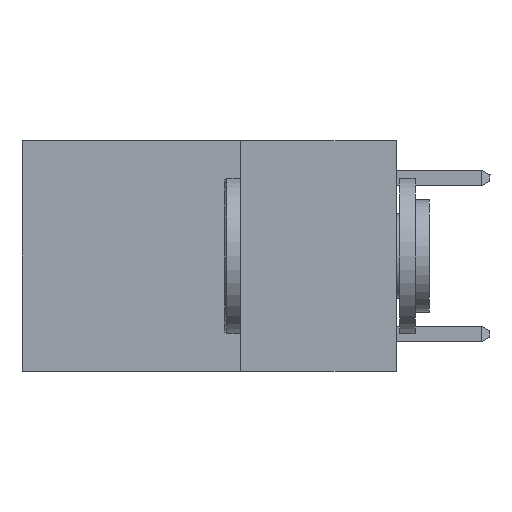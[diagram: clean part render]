
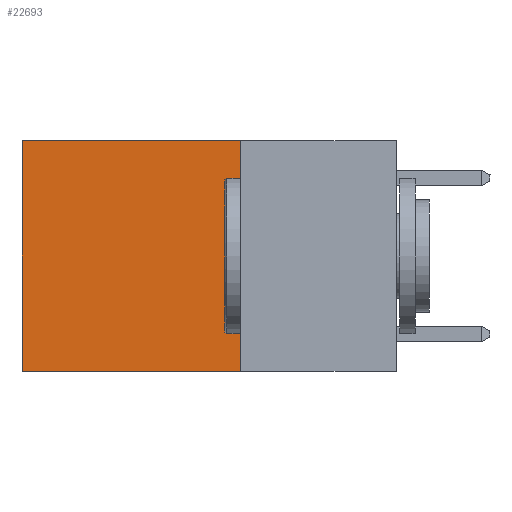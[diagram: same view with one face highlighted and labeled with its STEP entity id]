
A CAD part, left-side view. The second image highlights one B-rep face of the part: STEP entity #22693.
In plain terms, the highlighted planar face has unit normal (-1, 0, 0).
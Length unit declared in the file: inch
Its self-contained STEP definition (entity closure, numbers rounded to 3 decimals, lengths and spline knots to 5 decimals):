
#64 = LINE ( 'NONE', #23165, #13467 ) ;
#494 = LINE ( 'NONE', #6190, #6192 ) ;
#1434 = DIRECTION ( 'NONE',  ( 1., 0., 0. ) ) ;
#1438 = CARTESIAN_POINT ( 'NONE',  ( 0.2625, 0.25, -0.37 ) ) ;
#2534 = EDGE_LOOP ( 'NONE', ( #8610, #15364, #21157, #10491 ) ) ;
#2859 = PLANE ( 'NONE',  #4128 ) ;
#3209 = CARTESIAN_POINT ( 'NONE',  ( 0.2625, 0.25, 0. ) ) ;
#3812 = LINE ( 'NONE', #18160, #12394 ) ;
#4128 = AXIS2_PLACEMENT_3D ( 'NONE', #3209, #1434, #8187 ) ;
#6190 = CARTESIAN_POINT ( 'NONE',  ( 0.2625, 0.25, 0. ) ) ;
#6192 = VECTOR ( 'NONE', #16680, 39.37008 ) ;
#7245 = DIRECTION ( 'NONE',  ( 0., 1., 0. ) ) ;
#7482 = EDGE_CURVE ( 'NONE', #9780, #17205, #17042, .T. ) ;
#8187 = DIRECTION ( 'NONE',  ( 0., 0., -1. ) ) ;
#8610 = ORIENTED_EDGE ( 'NONE', *, *, #7482, .T. ) ;
#9780 = VERTEX_POINT ( 'NONE', #21618 ) ;
#10418 = FACE_OUTER_BOUND ( 'NONE', #2534, .T. ) ;
#10491 = ORIENTED_EDGE ( 'NONE', *, *, #22765, .T. ) ;
#11416 = CARTESIAN_POINT ( 'NONE',  ( 0.2625, 0.6, 0. ) ) ;
#12394 = VECTOR ( 'NONE', #7245, 39.37008 ) ;
#13327 = EDGE_CURVE ( 'NONE', #20105, #13596, #494, .T. ) ;
#13467 = VECTOR ( 'NONE', #19700, 39.37008 ) ;
#13541 = CARTESIAN_POINT ( 'NONE',  ( 0.2625, 0.6, -0.37 ) ) ;
#13596 = VERTEX_POINT ( 'NONE', #1438 ) ;
#15364 = ORIENTED_EDGE ( 'NONE', *, *, #22854, .F. ) ;
#16579 = VECTOR ( 'NONE', #16937, 39.37008 ) ;
#16680 = DIRECTION ( 'NONE',  ( 0., 0., -1. ) ) ;
#16937 = DIRECTION ( 'NONE',  ( 0., 0., -1. ) ) ;
#17042 = LINE ( 'NONE', #11416, #16579 ) ;
#17205 = VERTEX_POINT ( 'NONE', #13541 ) ;
#18160 = CARTESIAN_POINT ( 'NONE',  ( 0.2625, 0.25, -0.37 ) ) ;
#19700 = DIRECTION ( 'NONE',  ( 0., 1., 0. ) ) ;
#20105 = VERTEX_POINT ( 'NONE', #21928 ) ;
#21157 = ORIENTED_EDGE ( 'NONE', *, *, #13327, .F. ) ;
#21618 = CARTESIAN_POINT ( 'NONE',  ( 0.2625, 0.6, 0. ) ) ;
#21928 = CARTESIAN_POINT ( 'NONE',  ( 0.2625, 0.25, 0. ) ) ;
#22693 = ADVANCED_FACE ( 'NONE', ( #10418 ), #2859, .F. ) ;
#22765 = EDGE_CURVE ( 'NONE', #20105, #9780, #64, .T. ) ;
#22854 = EDGE_CURVE ( 'NONE', #13596, #17205, #3812, .T. ) ;
#23165 = CARTESIAN_POINT ( 'NONE',  ( 0.2625, 0.25, 0. ) ) ;
